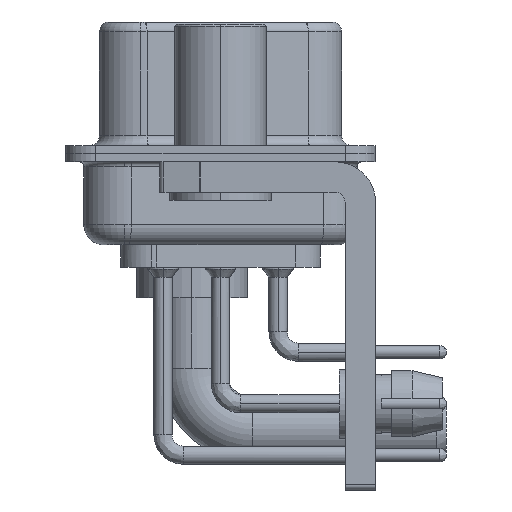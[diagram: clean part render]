
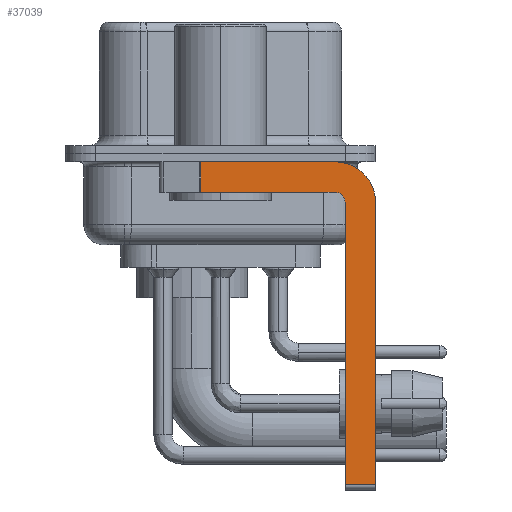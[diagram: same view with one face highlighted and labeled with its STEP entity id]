
A CAD part, left-side view. The second image highlights one B-rep face of the part: STEP entity #37039.
In plain terms, the highlighted planar face has unit normal (-1, 0, 0).
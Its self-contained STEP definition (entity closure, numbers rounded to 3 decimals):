
#319 = VERTEX_POINT ( 'NONE', #1232 ) ;
#446 = DIRECTION ( 'NONE',  ( 0., 0., -1. ) ) ;
#450 = DIRECTION ( 'NONE',  ( 1., 0., 0. ) ) ;
#1232 = CARTESIAN_POINT ( 'NONE',  ( -2.9, 0.978, -0.4 ) ) ;
#1514 = EDGE_CURVE ( 'NONE', #319, #10578, #14596, .T. ) ;
#2063 = ORIENTED_EDGE ( 'NONE', *, *, #27923, .F. ) ;
#2198 = DIRECTION ( 'NONE',  ( 0., -1., 0. ) ) ;
#3443 = VECTOR ( 'NONE', #2198, 1000. ) ;
#5226 = EDGE_CURVE ( 'NONE', #319, #37559, #29745, .T. ) ;
#5519 = CARTESIAN_POINT ( 'NONE',  ( -2.9, -6.15, -16.35 ) ) ;
#6430 = CARTESIAN_POINT ( 'NONE',  ( -2.9, -5.65, -2.4 ) ) ;
#6712 = VECTOR ( 'NONE', #21238, 1000. ) ;
#6733 = EDGE_LOOP ( 'NONE', ( #33428, #7326, #28664, #34645, #18798, #18178, #2063, #39314 ) ) ;
#7326 = ORIENTED_EDGE ( 'NONE', *, *, #1514, .T. ) ;
#7495 = EDGE_CURVE ( 'NONE', #37559, #33264, #24248, .T. ) ;
#8046 = CARTESIAN_POINT ( 'NONE',  ( -2.9, -6.15, -16.6 ) ) ;
#8339 = EDGE_CURVE ( 'NONE', #34628, #26185, #33923, .T. ) ;
#8846 = CARTESIAN_POINT ( 'NONE',  ( -2.9, -5.65, -16.35 ) ) ;
#9323 = CARTESIAN_POINT ( 'NONE',  ( -2.9, -5.65, -2.4 ) ) ;
#9473 = CARTESIAN_POINT ( 'NONE',  ( -2.9, -7.65, -16.35 ) ) ;
#10578 = VERTEX_POINT ( 'NONE', #39023 ) ;
#12726 = DIRECTION ( 'NONE',  ( 0., 0., -1. ) ) ;
#14596 = LINE ( 'NONE', #20262, #21844 ) ;
#14719 = FACE_OUTER_BOUND ( 'NONE', #6733, .T. ) ;
#15375 = VECTOR ( 'NONE', #29317, 1000. ) ;
#17042 = LINE ( 'NONE', #8046, #15375 ) ;
#17334 = EDGE_CURVE ( 'NONE', #26185, #10578, #33521, .T. ) ;
#17875 = DIRECTION ( 'NONE',  ( -1., 0., 0. ) ) ;
#18178 = ORIENTED_EDGE ( 'NONE', *, *, #35282, .T. ) ;
#18555 = CARTESIAN_POINT ( 'NONE',  ( -2.9, -7.65, -2.4 ) ) ;
#18597 = CARTESIAN_POINT ( 'NONE',  ( -2.9, -5.65, -1.9 ) ) ;
#18798 = ORIENTED_EDGE ( 'NONE', *, *, #25385, .F. ) ;
#18855 = CARTESIAN_POINT ( 'NONE',  ( -2.9, -5.65, -0.4 ) ) ;
#18951 = LINE ( 'NONE', #18555, #39359 ) ;
#19689 = AXIS2_PLACEMENT_3D ( 'NONE', #6430, #17875, #30144 ) ;
#20262 = CARTESIAN_POINT ( 'NONE',  ( -2.9, 0.978, -1.9 ) ) ;
#20914 = DIRECTION ( 'NONE',  ( 0., -1., 0. ) ) ;
#21238 = DIRECTION ( 'NONE',  ( 0., 1., 0. ) ) ;
#21844 = VECTOR ( 'NONE', #24075, 1000. ) ;
#23271 = AXIS2_PLACEMENT_3D ( 'NONE', #29826, #26616, #39506 ) ;
#24075 = DIRECTION ( 'NONE',  ( 0., 0., -1. ) ) ;
#24248 = CIRCLE ( 'NONE', #25530, 2. ) ;
#25385 = EDGE_CURVE ( 'NONE', #31762, #34628, #17042, .T. ) ;
#25530 = AXIS2_PLACEMENT_3D ( 'NONE', #9323, #450, #12726 ) ;
#26185 = VERTEX_POINT ( 'NONE', #18597 ) ;
#26616 = DIRECTION ( 'NONE',  ( 1., 0., 0. ) ) ;
#26950 = LINE ( 'NONE', #8846, #38671 ) ;
#27221 = PLANE ( 'NONE',  #23271 ) ;
#27881 = CARTESIAN_POINT ( 'NONE',  ( -2.9, -5.65, -1.9 ) ) ;
#27923 = EDGE_CURVE ( 'NONE', #33264, #33746, #18951, .T. ) ;
#28021 = CARTESIAN_POINT ( 'NONE',  ( -2.9, -7.65, -2.4 ) ) ;
#28664 = ORIENTED_EDGE ( 'NONE', *, *, #17334, .F. ) ;
#29317 = DIRECTION ( 'NONE',  ( 0., 0., 1. ) ) ;
#29530 = CARTESIAN_POINT ( 'NONE',  ( -2.9, 3., -0.4 ) ) ;
#29745 = LINE ( 'NONE', #29530, #3443 ) ;
#29826 = CARTESIAN_POINT ( 'NONE',  ( -2.9, -5.65, -2.4 ) ) ;
#30144 = DIRECTION ( 'NONE',  ( 0., 0., 1. ) ) ;
#31762 = VERTEX_POINT ( 'NONE', #5519 ) ;
#33264 = VERTEX_POINT ( 'NONE', #28021 ) ;
#33428 = ORIENTED_EDGE ( 'NONE', *, *, #5226, .F. ) ;
#33521 = LINE ( 'NONE', #27881, #6712 ) ;
#33746 = VERTEX_POINT ( 'NONE', #9473 ) ;
#33923 = CIRCLE ( 'NONE', #19689, 0.5 ) ;
#34517 = CARTESIAN_POINT ( 'NONE',  ( -2.9, -6.15, -2.4 ) ) ;
#34628 = VERTEX_POINT ( 'NONE', #34517 ) ;
#34645 = ORIENTED_EDGE ( 'NONE', *, *, #8339, .F. ) ;
#35282 = EDGE_CURVE ( 'NONE', #31762, #33746, #26950, .T. ) ;
#37039 = ADVANCED_FACE ( 'NONE', ( #14719 ), #27221, .F. ) ;
#37559 = VERTEX_POINT ( 'NONE', #18855 ) ;
#38671 = VECTOR ( 'NONE', #20914, 1000. ) ;
#39023 = CARTESIAN_POINT ( 'NONE',  ( -2.9, 0.978, -1.9 ) ) ;
#39314 = ORIENTED_EDGE ( 'NONE', *, *, #7495, .F. ) ;
#39359 = VECTOR ( 'NONE', #446, 1000. ) ;
#39506 = DIRECTION ( 'NONE',  ( 0., 0., -1. ) ) ;
